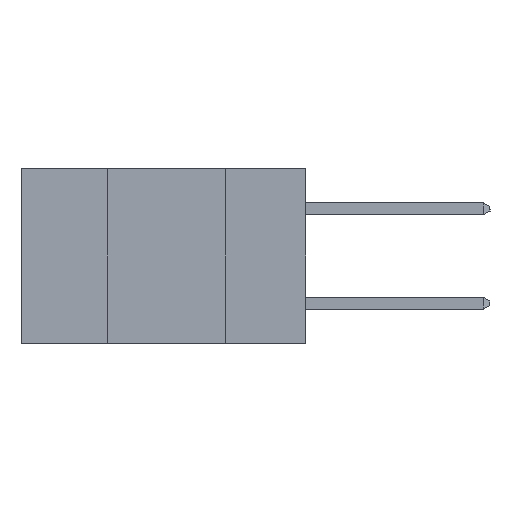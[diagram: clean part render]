
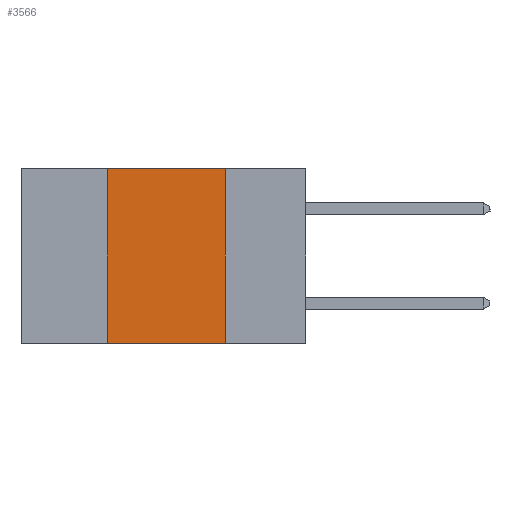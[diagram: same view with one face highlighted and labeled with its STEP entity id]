
A CAD part, left-side view. The second image highlights one B-rep face of the part: STEP entity #3566.
In plain terms, the highlighted planar face has unit normal (-1, 0, 0).
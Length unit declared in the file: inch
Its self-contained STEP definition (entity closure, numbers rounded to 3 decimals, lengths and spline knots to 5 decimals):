
#591 = VERTEX_POINT ( 'NONE', #3049 ) ;
#699 = DIRECTION ( 'NONE',  ( 0., 0., -1. ) ) ;
#746 = DIRECTION ( 'NONE',  ( 1., 0., 0. ) ) ;
#857 = PLANE ( 'NONE',  #22596 ) ;
#2416 = CARTESIAN_POINT ( 'NONE',  ( 0., 0.6, 0. ) ) ;
#3049 = CARTESIAN_POINT ( 'NONE',  ( 0., 0.42, -0.37 ) ) ;
#3159 = EDGE_CURVE ( 'NONE', #591, #11408, #9269, .T. ) ;
#3270 = ORIENTED_EDGE ( 'NONE', *, *, #4390, .T. ) ;
#3566 = ADVANCED_FACE ( 'NONE', ( #15827 ), #857, .F. ) ;
#3956 = DIRECTION ( 'NONE',  ( 0., -1., 0. ) ) ;
#4065 = LINE ( 'NONE', #19829, #22304 ) ;
#4338 = VECTOR ( 'NONE', #4828, 39.37008 ) ;
#4390 = EDGE_CURVE ( 'NONE', #591, #13111, #21113, .T. ) ;
#4805 = EDGE_LOOP ( 'NONE', ( #7878, #17578, #20408, #3270 ) ) ;
#4828 = DIRECTION ( 'NONE',  ( 0., 0., 1. ) ) ;
#7878 = ORIENTED_EDGE ( 'NONE', *, *, #20003, .F. ) ;
#8667 = VECTOR ( 'NONE', #3956, 39.37008 ) ;
#8783 = VERTEX_POINT ( 'NONE', #10484 ) ;
#9269 = LINE ( 'NONE', #17757, #4338 ) ;
#10448 = CARTESIAN_POINT ( 'NONE',  ( 0., 0.17, -0.37 ) ) ;
#10483 = DIRECTION ( 'NONE',  ( 0., -1., 0. ) ) ;
#10484 = CARTESIAN_POINT ( 'NONE',  ( 0., 0.17, 0. ) ) ;
#11408 = VERTEX_POINT ( 'NONE', #16872 ) ;
#12069 = VECTOR ( 'NONE', #10483, 39.37008 ) ;
#13111 = VERTEX_POINT ( 'NONE', #10448 ) ;
#15186 = EDGE_CURVE ( 'NONE', #11408, #8783, #17210, .T. ) ;
#15827 = FACE_OUTER_BOUND ( 'NONE', #4805, .T. ) ;
#16292 = DIRECTION ( 'NONE',  ( 0., 0., -1. ) ) ;
#16789 = CARTESIAN_POINT ( 'NONE',  ( 0., 0.6, 0. ) ) ;
#16872 = CARTESIAN_POINT ( 'NONE',  ( 0., 0.42, 0. ) ) ;
#17210 = LINE ( 'NONE', #16789, #8667 ) ;
#17578 = ORIENTED_EDGE ( 'NONE', *, *, #15186, .F. ) ;
#17757 = CARTESIAN_POINT ( 'NONE',  ( 0., 0.42, 0. ) ) ;
#19829 = CARTESIAN_POINT ( 'NONE',  ( 0., 0.17, 0. ) ) ;
#20003 = EDGE_CURVE ( 'NONE', #8783, #13111, #4065, .T. ) ;
#20408 = ORIENTED_EDGE ( 'NONE', *, *, #3159, .F. ) ;
#21113 = LINE ( 'NONE', #21323, #12069 ) ;
#21323 = CARTESIAN_POINT ( 'NONE',  ( 0., 0.6, -0.37 ) ) ;
#22304 = VECTOR ( 'NONE', #16292, 39.37008 ) ;
#22596 = AXIS2_PLACEMENT_3D ( 'NONE', #2416, #746, #699 ) ;
